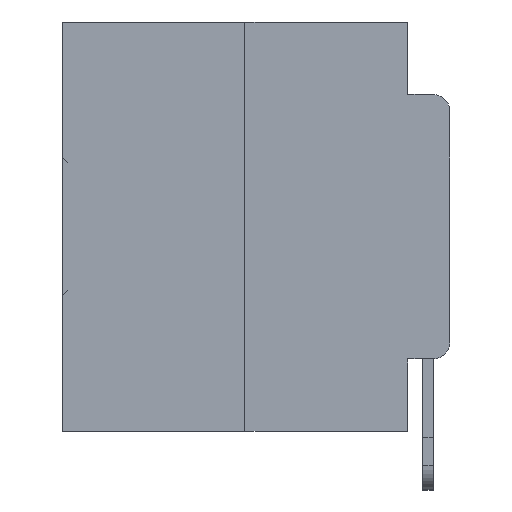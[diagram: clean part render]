
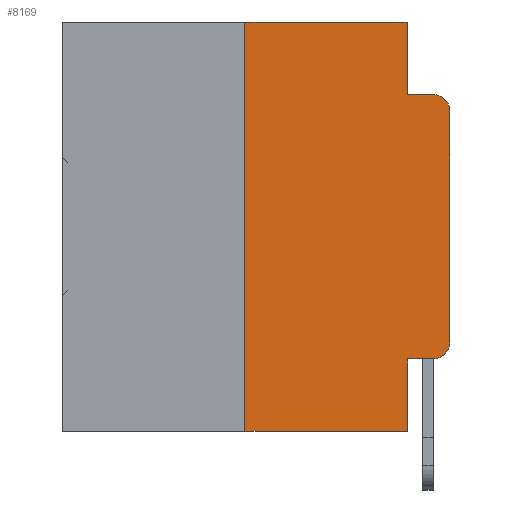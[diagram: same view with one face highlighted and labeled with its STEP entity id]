
A CAD part, left-side view. The second image highlights one B-rep face of the part: STEP entity #8169.
In plain terms, the highlighted planar face has unit normal (-1, 0, 0).
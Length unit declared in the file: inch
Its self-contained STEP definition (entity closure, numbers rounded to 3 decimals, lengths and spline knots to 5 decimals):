
#65 = CARTESIAN_POINT ( 'NONE',  ( 0., 0.051, 0. ) ) ;
#897 = EDGE_CURVE ( 'NONE', #31406, #11965, #18365, .T. ) ;
#954 = CARTESIAN_POINT ( 'NONE',  ( 0., 0.473, 0. ) ) ;
#1160 = VECTOR ( 'NONE', #2976, 39.37008 ) ;
#1640 = CIRCLE ( 'NONE', #20424, 0.02 ) ;
#1854 = VECTOR ( 'NONE', #30953, 39.37008 ) ;
#2568 = CARTESIAN_POINT ( 'NONE',  ( 0., 0.051, 0. ) ) ;
#2976 = DIRECTION ( 'NONE',  ( 0., 0., -1. ) ) ;
#3392 = LINE ( 'NONE', #954, #30394 ) ;
#3804 = DIRECTION ( 'NONE',  ( 0., -1., 0. ) ) ;
#3997 = CIRCLE ( 'NONE', #23232, 0.02 ) ;
#4557 = PLANE ( 'NONE',  #29742 ) ;
#4893 = EDGE_CURVE ( 'NONE', #31406, #21837, #9184, .T. ) ;
#5001 = ORIENTED_EDGE ( 'NONE', *, *, #5391, .T. ) ;
#5231 = LINE ( 'NONE', #32024, #24181 ) ;
#5283 = DIRECTION ( 'NONE',  ( -1., 0., 0. ) ) ;
#5329 = VERTEX_POINT ( 'NONE', #33224 ) ;
#5391 = EDGE_CURVE ( 'NONE', #20223, #5329, #16304, .T. ) ;
#5762 = ORIENTED_EDGE ( 'NONE', *, *, #26773, .F. ) ;
#5768 = ORIENTED_EDGE ( 'NONE', *, *, #4893, .T. ) ;
#6508 = CARTESIAN_POINT ( 'NONE',  ( 0., 0.02, -0.0885 ) ) ;
#7308 = DIRECTION ( 'NONE',  ( 1., 0., 0. ) ) ;
#7985 = VERTEX_POINT ( 'NONE', #6508 ) ;
#8169 = ADVANCED_FACE ( 'NONE', ( #24522 ), #4557, .F. ) ;
#9165 = VERTEX_POINT ( 'NONE', #10496 ) ;
#9184 = LINE ( 'NONE', #10322, #22643 ) ;
#9647 = EDGE_CURVE ( 'NONE', #5329, #23799, #3997, .T. ) ;
#10322 = CARTESIAN_POINT ( 'NONE',  ( 0., 0.473, -0.5 ) ) ;
#10496 = CARTESIAN_POINT ( 'NONE',  ( 0., 0.051, -0.0885 ) ) ;
#10918 = DIRECTION ( 'NONE',  ( 0., -1., 0. ) ) ;
#11195 = VECTOR ( 'NONE', #27761, 39.37008 ) ;
#11965 = VERTEX_POINT ( 'NONE', #12923 ) ;
#12354 = CARTESIAN_POINT ( 'NONE',  ( 0., 0., 0. ) ) ;
#12923 = CARTESIAN_POINT ( 'NONE',  ( 0., 0.25, 0. ) ) ;
#12959 = DIRECTION ( 'NONE',  ( 0., -1., 0. ) ) ;
#13233 = EDGE_CURVE ( 'NONE', #20223, #21837, #5231, .T. ) ;
#13756 = ORIENTED_EDGE ( 'NONE', *, *, #13233, .F. ) ;
#14138 = EDGE_CURVE ( 'NONE', #28792, #7985, #1640, .T. ) ;
#14162 = DIRECTION ( 'NONE',  ( -1., 0., 0. ) ) ;
#14942 = ORIENTED_EDGE ( 'NONE', *, *, #897, .F. ) ;
#15263 = CARTESIAN_POINT ( 'NONE',  ( 0., 0.473, 0. ) ) ;
#15458 = EDGE_CURVE ( 'NONE', #23799, #28792, #17896, .T. ) ;
#15660 = LINE ( 'NONE', #65, #1160 ) ;
#15835 = ORIENTED_EDGE ( 'NONE', *, *, #15458, .T. ) ;
#16304 = LINE ( 'NONE', #28269, #1854 ) ;
#16875 = EDGE_LOOP ( 'NONE', ( #15835, #20163, #33192, #23551, #5762, #14942, #5768, #13756, #5001, #35042 ) ) ;
#17896 = LINE ( 'NONE', #12354, #32140 ) ;
#18365 = LINE ( 'NONE', #19672, #11195 ) ;
#19672 = CARTESIAN_POINT ( 'NONE',  ( 0., 0.25, 0. ) ) ;
#20163 = ORIENTED_EDGE ( 'NONE', *, *, #14138, .T. ) ;
#20223 = VERTEX_POINT ( 'NONE', #23363 ) ;
#20424 = AXIS2_PLACEMENT_3D ( 'NONE', #30308, #14162, #32927 ) ;
#21407 = CARTESIAN_POINT ( 'NONE',  ( 0., 0.02, -0.3915 ) ) ;
#21837 = VERTEX_POINT ( 'NONE', #34308 ) ;
#22643 = VECTOR ( 'NONE', #12959, 39.37008 ) ;
#23232 = AXIS2_PLACEMENT_3D ( 'NONE', #21407, #5283, #24106 ) ;
#23363 = CARTESIAN_POINT ( 'NONE',  ( 0., 0.051, -0.4115 ) ) ;
#23551 = ORIENTED_EDGE ( 'NONE', *, *, #26550, .F. ) ;
#23799 = VERTEX_POINT ( 'NONE', #31338 ) ;
#24003 = VERTEX_POINT ( 'NONE', #2568 ) ;
#24106 = DIRECTION ( 'NONE',  ( 0., 0., -1. ) ) ;
#24181 = VECTOR ( 'NONE', #29498, 39.37008 ) ;
#24522 = FACE_OUTER_BOUND ( 'NONE', #16875, .T. ) ;
#24569 = VECTOR ( 'NONE', #10918, 39.37008 ) ;
#25417 = EDGE_CURVE ( 'NONE', #9165, #7985, #31659, .T. ) ;
#26105 = DIRECTION ( 'NONE',  ( 0., 0., -1. ) ) ;
#26431 = CARTESIAN_POINT ( 'NONE',  ( 0., 0., -0.1085 ) ) ;
#26550 = EDGE_CURVE ( 'NONE', #24003, #9165, #15660, .T. ) ;
#26773 = EDGE_CURVE ( 'NONE', #11965, #24003, #3392, .T. ) ;
#27039 = CARTESIAN_POINT ( 'NONE',  ( 0., 0.051, -0.0885 ) ) ;
#27761 = DIRECTION ( 'NONE',  ( 0., 0., 1. ) ) ;
#28269 = CARTESIAN_POINT ( 'NONE',  ( 0., 0.051, -0.4115 ) ) ;
#28792 = VERTEX_POINT ( 'NONE', #26431 ) ;
#29498 = DIRECTION ( 'NONE',  ( 0., 0., -1. ) ) ;
#29742 = AXIS2_PLACEMENT_3D ( 'NONE', #15263, #7308, #26105 ) ;
#30308 = CARTESIAN_POINT ( 'NONE',  ( 0., 0.02, -0.1085 ) ) ;
#30394 = VECTOR ( 'NONE', #3804, 39.37008 ) ;
#30953 = DIRECTION ( 'NONE',  ( 0., -1., 0. ) ) ;
#31177 = DIRECTION ( 'NONE',  ( 0., 0., 1. ) ) ;
#31338 = CARTESIAN_POINT ( 'NONE',  ( 0., 0., -0.3915 ) ) ;
#31351 = CARTESIAN_POINT ( 'NONE',  ( 0., 0.25, -0.5 ) ) ;
#31406 = VERTEX_POINT ( 'NONE', #31351 ) ;
#31659 = LINE ( 'NONE', #27039, #24569 ) ;
#32024 = CARTESIAN_POINT ( 'NONE',  ( 0., 0.051, 0. ) ) ;
#32140 = VECTOR ( 'NONE', #31177, 39.37008 ) ;
#32927 = DIRECTION ( 'NONE',  ( 0., 0., -1. ) ) ;
#33192 = ORIENTED_EDGE ( 'NONE', *, *, #25417, .F. ) ;
#33224 = CARTESIAN_POINT ( 'NONE',  ( 0., 0.02, -0.4115 ) ) ;
#34308 = CARTESIAN_POINT ( 'NONE',  ( 0., 0.051, -0.5 ) ) ;
#35042 = ORIENTED_EDGE ( 'NONE', *, *, #9647, .T. ) ;
